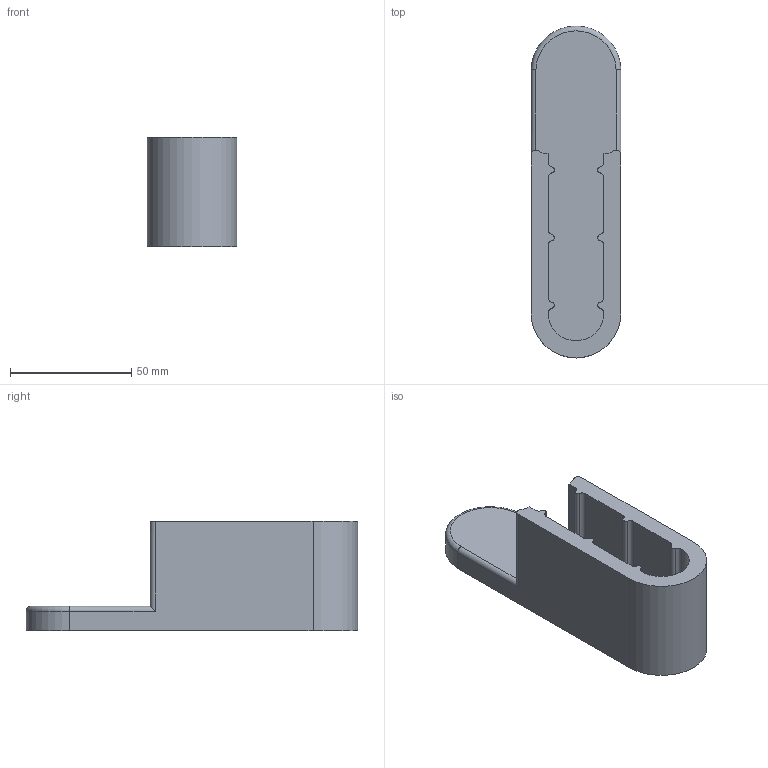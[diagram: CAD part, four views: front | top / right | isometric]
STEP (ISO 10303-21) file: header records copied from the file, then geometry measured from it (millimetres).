
FILE_DESCRIPTION (( 'STEP AP214' ), '1' );
FILE_NAME ('Rifle_Stock_Cap_1.step', '2019-12-18T03:08:35', ( '' ), ( '' ), 'SwSTEP 2.0', 'SolidWorks 2019', '' );
FILE_SCHEMA (( 'AUTOMOTIVE_DESIGN' ));
Length unit declared in the file: millimetre
Products named in the file (1): Rifle_Stock_Cap_1
Bounding box: 37.13 x 137.04 x 45 mm (x, y, z)
Volume: 93020.8 mm3; surface area: 26526.2 mm2
Topology: 1 solids, 1 shells, 47 faces, 127 edges, 84 vertices
Faces by surface type: cylinder 33, plane 13, torus 1
Entity records: 1566 total; most frequent: CARTESIAN_POINT 293, DIRECTION 282, ORIENTED_EDGE 254, EDGE_CURVE 127, AXIS2_PLACEMENT_3D 111, VERTEX_POINT 84, CIRCLE 63, VECTOR 60
